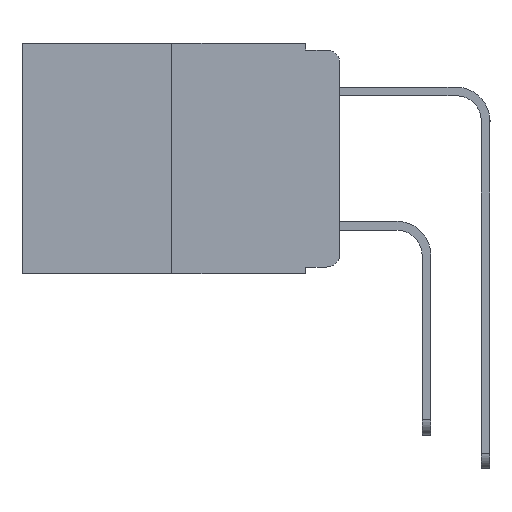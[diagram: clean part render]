
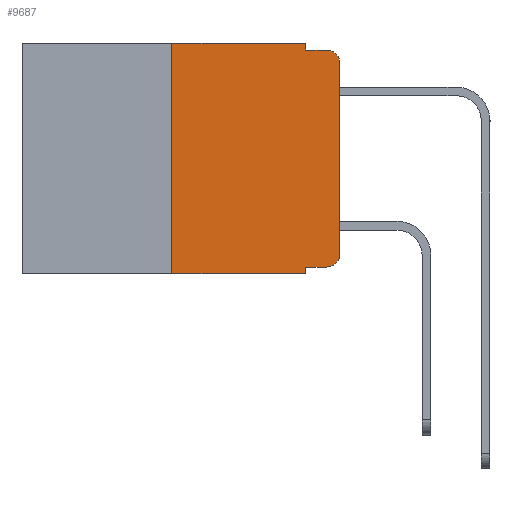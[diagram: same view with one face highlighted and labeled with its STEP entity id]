
A CAD part, left-side view. The second image highlights one B-rep face of the part: STEP entity #9687.
In plain terms, the highlighted planar face has unit normal (-1, 0, 0).
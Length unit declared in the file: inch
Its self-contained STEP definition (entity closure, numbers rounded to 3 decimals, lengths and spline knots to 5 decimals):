
#47 = VECTOR ( 'NONE', #7215, 39.37008 ) ;
#419 = VERTEX_POINT ( 'NONE', #18276 ) ;
#616 = LINE ( 'NONE', #1595, #47 ) ;
#685 = DIRECTION ( 'NONE',  ( 0., -1., 0. ) ) ;
#1046 = ORIENTED_EDGE ( 'NONE', *, *, #18261, .T. ) ;
#1312 = CARTESIAN_POINT ( 'NONE',  ( 0., 0.051, -0.01 ) ) ;
#1425 = DIRECTION ( 'NONE',  ( -1., 0., 0. ) ) ;
#1595 = CARTESIAN_POINT ( 'NONE',  ( 0., 0.25, 0. ) ) ;
#2528 = VERTEX_POINT ( 'NONE', #17176 ) ;
#2804 = LINE ( 'NONE', #16293, #11833 ) ;
#2844 = CARTESIAN_POINT ( 'NONE',  ( 0., 0.02, -0.01 ) ) ;
#2869 = AXIS2_PLACEMENT_3D ( 'NONE', #11630, #1425, #13266 ) ;
#2942 = ORIENTED_EDGE ( 'NONE', *, *, #17237, .T. ) ;
#3340 = CIRCLE ( 'NONE', #5153, 0.02 ) ;
#3440 = VERTEX_POINT ( 'NONE', #10766 ) ;
#3555 = DIRECTION ( 'NONE',  ( 1., 0., 0. ) ) ;
#4001 = EDGE_CURVE ( 'NONE', #11834, #5143, #616, .T. ) ;
#4026 = ORIENTED_EDGE ( 'NONE', *, *, #4001, .F. ) ;
#4882 = LINE ( 'NONE', #4954, #12797 ) ;
#4886 = CARTESIAN_POINT ( 'NONE',  ( 0., 0.02, -0.03 ) ) ;
#4954 = CARTESIAN_POINT ( 'NONE',  ( 0., 0., 0. ) ) ;
#5074 = FACE_OUTER_BOUND ( 'NONE', #13196, .T. ) ;
#5143 = VERTEX_POINT ( 'NONE', #5828 ) ;
#5153 = AXIS2_PLACEMENT_3D ( 'NONE', #4886, #16405, #6592 ) ;
#5824 = CARTESIAN_POINT ( 'NONE',  ( 0., 0.25, -0.343 ) ) ;
#5828 = CARTESIAN_POINT ( 'NONE',  ( 0., 0.25, 0. ) ) ;
#5972 = CARTESIAN_POINT ( 'NONE',  ( 0., 0.051, 0. ) ) ;
#6532 = CARTESIAN_POINT ( 'NONE',  ( 0., 0.473, 0. ) ) ;
#6592 = DIRECTION ( 'NONE',  ( 0., 0., -1. ) ) ;
#6676 = DIRECTION ( 'NONE',  ( 0., 0., 1. ) ) ;
#6767 = AXIS2_PLACEMENT_3D ( 'NONE', #18262, #3555, #19868 ) ;
#6807 = VERTEX_POINT ( 'NONE', #2844 ) ;
#7031 = EDGE_CURVE ( 'NONE', #20681, #20842, #20860, .T. ) ;
#7215 = DIRECTION ( 'NONE',  ( 0., 0., 1. ) ) ;
#8186 = EDGE_CURVE ( 'NONE', #13701, #15877, #4882, .T. ) ;
#8279 = DIRECTION ( 'NONE',  ( 0., -1., 0. ) ) ;
#8463 = CARTESIAN_POINT ( 'NONE',  ( 0., 0.051, -0.01 ) ) ;
#8546 = DIRECTION ( 'NONE',  ( 0., 0., -1. ) ) ;
#8696 = VECTOR ( 'NONE', #8546, 39.37008 ) ;
#9119 = ORIENTED_EDGE ( 'NONE', *, *, #9610, .T. ) ;
#9610 = EDGE_CURVE ( 'NONE', #11834, #2528, #19080, .T. ) ;
#9687 = ADVANCED_FACE ( 'NONE', ( #5074 ), #16774, .F. ) ;
#10209 = DIRECTION ( 'NONE',  ( 0., -1., 0. ) ) ;
#10231 = VECTOR ( 'NONE', #685, 39.37008 ) ;
#10766 = CARTESIAN_POINT ( 'NONE',  ( 0., 0.051, -0.333 ) ) ;
#11630 = CARTESIAN_POINT ( 'NONE',  ( 0., 0.02, -0.313 ) ) ;
#11810 = DIRECTION ( 'NONE',  ( 0., -1., 0. ) ) ;
#11833 = VECTOR ( 'NONE', #17881, 39.37008 ) ;
#11834 = VERTEX_POINT ( 'NONE', #5824 ) ;
#11862 = CARTESIAN_POINT ( 'NONE',  ( 0., 0.473, -0.343 ) ) ;
#11965 = ORIENTED_EDGE ( 'NONE', *, *, #18542, .F. ) ;
#12474 = ORIENTED_EDGE ( 'NONE', *, *, #13326, .F. ) ;
#12797 = VECTOR ( 'NONE', #6676, 39.37008 ) ;
#13196 = EDGE_LOOP ( 'NONE', ( #15693, #2942, #11965, #16180, #12474, #4026, #9119, #17664, #1046, #18611 ) ) ;
#13266 = DIRECTION ( 'NONE',  ( 0., 0., -1. ) ) ;
#13286 = VECTOR ( 'NONE', #11810, 39.37008 ) ;
#13326 = EDGE_CURVE ( 'NONE', #5143, #20681, #20068, .T. ) ;
#13701 = VERTEX_POINT ( 'NONE', #20321 ) ;
#14942 = VECTOR ( 'NONE', #10209, 39.37008 ) ;
#15693 = ORIENTED_EDGE ( 'NONE', *, *, #8186, .T. ) ;
#15703 = CARTESIAN_POINT ( 'NONE',  ( 0., 0.051, -0.333 ) ) ;
#15877 = VERTEX_POINT ( 'NONE', #21293 ) ;
#16180 = ORIENTED_EDGE ( 'NONE', *, *, #7031, .F. ) ;
#16293 = CARTESIAN_POINT ( 'NONE',  ( 0., 0.051, 0. ) ) ;
#16405 = DIRECTION ( 'NONE',  ( -1., 0., 0. ) ) ;
#16774 = PLANE ( 'NONE',  #6767 ) ;
#17176 = CARTESIAN_POINT ( 'NONE',  ( 0., 0.051, -0.343 ) ) ;
#17229 = EDGE_CURVE ( 'NONE', #419, #13701, #20171, .T. ) ;
#17237 = EDGE_CURVE ( 'NONE', #15877, #6807, #3340, .T. ) ;
#17459 = LINE ( 'NONE', #8463, #13286 ) ;
#17664 = ORIENTED_EDGE ( 'NONE', *, *, #19026, .F. ) ;
#17881 = DIRECTION ( 'NONE',  ( 0., 0., -1. ) ) ;
#18159 = CARTESIAN_POINT ( 'NONE',  ( 0., 0.051, 0. ) ) ;
#18261 = EDGE_CURVE ( 'NONE', #3440, #419, #18664, .T. ) ;
#18262 = CARTESIAN_POINT ( 'NONE',  ( 0., 0.473, 0. ) ) ;
#18276 = CARTESIAN_POINT ( 'NONE',  ( 0., 0.02, -0.333 ) ) ;
#18542 = EDGE_CURVE ( 'NONE', #20842, #6807, #17459, .T. ) ;
#18611 = ORIENTED_EDGE ( 'NONE', *, *, #17229, .T. ) ;
#18664 = LINE ( 'NONE', #15703, #10231 ) ;
#19026 = EDGE_CURVE ( 'NONE', #3440, #2528, #2804, .T. ) ;
#19080 = LINE ( 'NONE', #11862, #14942 ) ;
#19577 = VECTOR ( 'NONE', #8279, 39.37008 ) ;
#19868 = DIRECTION ( 'NONE',  ( 0., 0., -1. ) ) ;
#20068 = LINE ( 'NONE', #6532, #19577 ) ;
#20171 = CIRCLE ( 'NONE', #2869, 0.02 ) ;
#20321 = CARTESIAN_POINT ( 'NONE',  ( 0., 0., -0.313 ) ) ;
#20681 = VERTEX_POINT ( 'NONE', #5972 ) ;
#20842 = VERTEX_POINT ( 'NONE', #1312 ) ;
#20860 = LINE ( 'NONE', #18159, #8696 ) ;
#21293 = CARTESIAN_POINT ( 'NONE',  ( 0., 0., -0.03 ) ) ;
